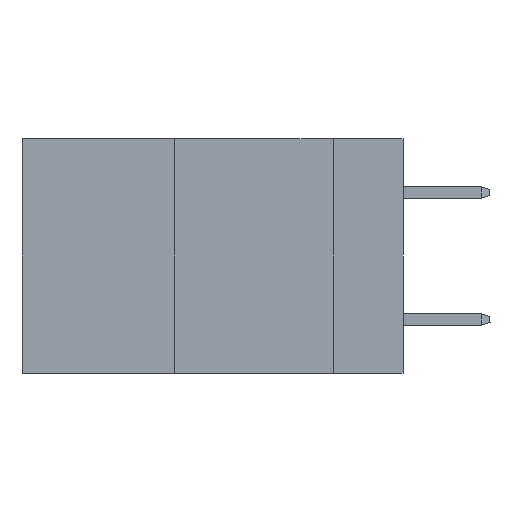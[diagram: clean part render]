
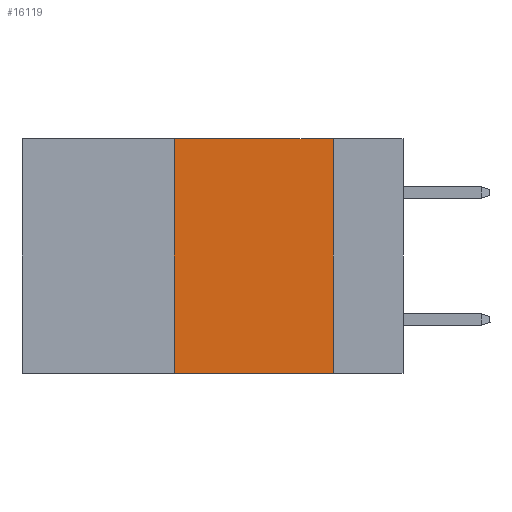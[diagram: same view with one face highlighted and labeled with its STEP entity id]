
A CAD part, left-side view. The second image highlights one B-rep face of the part: STEP entity #16119.
In plain terms, the highlighted planar face has unit normal (-1, 0, 0).
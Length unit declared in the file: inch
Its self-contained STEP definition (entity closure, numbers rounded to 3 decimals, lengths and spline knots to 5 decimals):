
#1023 = VECTOR ( 'NONE', #15711, 39.37008 ) ;
#1292 = VERTEX_POINT ( 'NONE', #5367 ) ;
#1342 = LINE ( 'NONE', #8760, #12663 ) ;
#1955 = DIRECTION ( 'NONE',  ( 1., 0., 0. ) ) ;
#2096 = VECTOR ( 'NONE', #17064, 39.37008 ) ;
#2896 = CARTESIAN_POINT ( 'NONE',  ( 0., 0.11, 0. ) ) ;
#3901 = DIRECTION ( 'NONE',  ( 0., 0., -1. ) ) ;
#5367 = CARTESIAN_POINT ( 'NONE',  ( 0., 0.36, 0. ) ) ;
#5984 = ORIENTED_EDGE ( 'NONE', *, *, #12033, .F. ) ;
#6927 = VERTEX_POINT ( 'NONE', #10026 ) ;
#7232 = ORIENTED_EDGE ( 'NONE', *, *, #17354, .T. ) ;
#8622 = ORIENTED_EDGE ( 'NONE', *, *, #14900, .F. ) ;
#8760 = CARTESIAN_POINT ( 'NONE',  ( 0., 0.36, 0. ) ) ;
#10026 = CARTESIAN_POINT ( 'NONE',  ( 0., 0.11, 0. ) ) ;
#10311 = DIRECTION ( 'NONE',  ( 0., 0., -1. ) ) ;
#11596 = EDGE_CURVE ( 'NONE', #1292, #6927, #11815, .T. ) ;
#11815 = LINE ( 'NONE', #19372, #1023 ) ;
#12033 = EDGE_CURVE ( 'NONE', #15488, #1292, #1342, .T. ) ;
#12049 = CARTESIAN_POINT ( 'NONE',  ( 0., 0.36, -0.37 ) ) ;
#12663 = VECTOR ( 'NONE', #23972, 39.37008 ) ;
#14900 = EDGE_CURVE ( 'NONE', #6927, #23441, #19573, .T. ) ;
#15488 = VERTEX_POINT ( 'NONE', #12049 ) ;
#15711 = DIRECTION ( 'NONE',  ( 0., -1., 0. ) ) ;
#16119 = ADVANCED_FACE ( 'NONE', ( #22535 ), #16692, .F. ) ;
#16692 = PLANE ( 'NONE',  #21880 ) ;
#17064 = DIRECTION ( 'NONE',  ( 0., -1., 0. ) ) ;
#17136 = ORIENTED_EDGE ( 'NONE', *, *, #11596, .F. ) ;
#17354 = EDGE_CURVE ( 'NONE', #15488, #23441, #21213, .T. ) ;
#18714 = VECTOR ( 'NONE', #10311, 39.37008 ) ;
#19372 = CARTESIAN_POINT ( 'NONE',  ( 0., 0.6, 0. ) ) ;
#19573 = LINE ( 'NONE', #2896, #18714 ) ;
#20579 = CARTESIAN_POINT ( 'NONE',  ( 0., 0.6, 0. ) ) ;
#21213 = LINE ( 'NONE', #22804, #2096 ) ;
#21880 = AXIS2_PLACEMENT_3D ( 'NONE', #20579, #1955, #3901 ) ;
#22535 = FACE_OUTER_BOUND ( 'NONE', #22883, .T. ) ;
#22663 = CARTESIAN_POINT ( 'NONE',  ( 0., 0.11, -0.37 ) ) ;
#22804 = CARTESIAN_POINT ( 'NONE',  ( 0., 0.6, -0.37 ) ) ;
#22883 = EDGE_LOOP ( 'NONE', ( #8622, #17136, #5984, #7232 ) ) ;
#23441 = VERTEX_POINT ( 'NONE', #22663 ) ;
#23972 = DIRECTION ( 'NONE',  ( 0., 0., 1. ) ) ;
